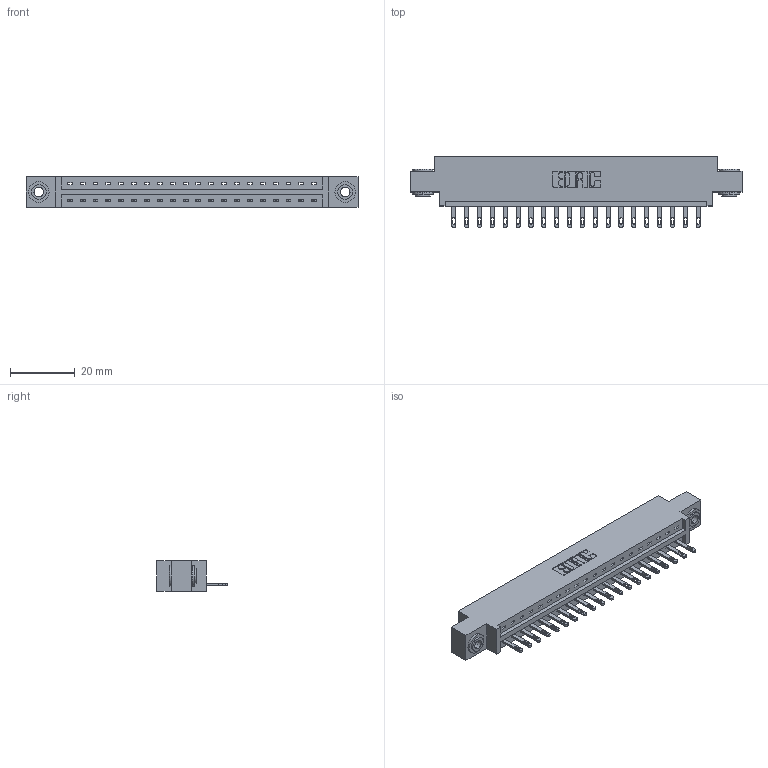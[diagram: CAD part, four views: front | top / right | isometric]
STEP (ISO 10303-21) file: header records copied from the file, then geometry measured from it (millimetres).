
FILE_DESCRIPTION (( 'STEP AP203' ), '1' );
FILE_NAME ('337-020-500-603.STEP', '2019-09-28T22:16:24', ( '' ), ( '' ), 'SwSTEP 2.0', 'SolidWorks 2016', '' );
FILE_SCHEMA (( 'CONFIG_CONTROL_DESIGN' ));
Length unit declared in the file: inch
Products named in the file (4): 337-020-500-603; 345-250-002_345-250-002-102; 345-292-001_345-293-100; 337 Part_0.170 Offset - 0.156 Dia-TH
Assembly tree (23 placements, depth 2):
  337-020-500-603
    337 Part_0.170 Offset - 0.156 Dia-TH
    345-292-001_345-293-100  x20
    345-250-002_345-250-002-102  x2
Bounding box: 102.26 x 21.85 x 9.4 mm (x, y, z)
Volume: 10267.2 mm3; surface area: 10863.4 mm2
Topology: 23 solids, 23 shells, 1316 faces, 3999 edges, 2662 vertices
Faces by surface type: plane 884, cylinder 424, cone 8
Entity records: 18424 total; most frequent: CARTESIAN_POINT 3185, ORIENTED_EDGE 3134, DIRECTION 2761, EDGE_CURVE 1567, LINE 1411, VECTOR 1411, VERTEX_POINT 1042, AXIS2_PLACEMENT_3D 675
